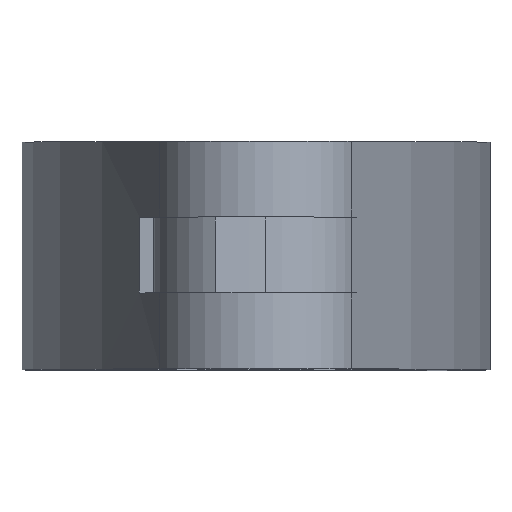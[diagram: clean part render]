
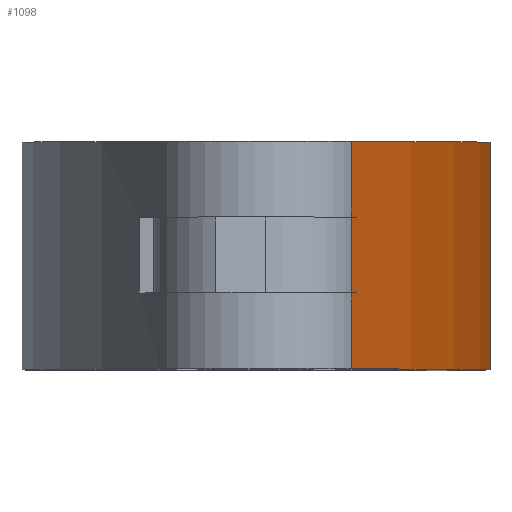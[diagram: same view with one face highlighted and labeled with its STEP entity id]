
A CAD part, top view. The second image highlights one B-rep face of the part: STEP entity #1098.
In plain terms, the highlighted cylindrical face has radius 200.536 mm (diameter 401.073 mm), a partial arc.
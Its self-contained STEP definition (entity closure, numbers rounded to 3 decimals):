
#106=FACE_OUTER_BOUND('',#176,.T.);
#176=EDGE_LOOP('',(#885,#886,#887,#888,#889,#890));
#229=LINE('',#1758,#317);
#251=LINE('',#1899,#339);
#256=LINE('',#1908,#344);
#257=LINE('',#1910,#345);
#317=VECTOR('',#1405,10.);
#339=VECTOR('',#1475,10.);
#344=VECTOR('',#1488,10.);
#345=VECTOR('',#1491,10.);
#398=CIRCLE('',#1170,200.536);
#406=CIRCLE('',#1181,200.536);
#469=VERTEX_POINT('',#1685);
#470=VERTEX_POINT('',#1687);
#479=VERTEX_POINT('',#1711);
#480=VERTEX_POINT('',#1713);
#493=VERTEX_POINT('',#1744);
#495=VERTEX_POINT('',#1752);
#573=EDGE_CURVE('',#470,#469,#398,.T.);
#586=EDGE_CURVE('',#479,#480,#406,.T.);
#608=EDGE_CURVE('',#493,#495,#229,.T.);
#641=EDGE_CURVE('',#495,#469,#251,.T.);
#646=EDGE_CURVE('',#480,#493,#256,.T.);
#647=EDGE_CURVE('',#479,#470,#257,.T.);
#885=ORIENTED_EDGE('',*,*,#586,.F.);
#886=ORIENTED_EDGE('',*,*,#647,.T.);
#887=ORIENTED_EDGE('',*,*,#573,.T.);
#888=ORIENTED_EDGE('',*,*,#641,.F.);
#889=ORIENTED_EDGE('',*,*,#608,.F.);
#890=ORIENTED_EDGE('',*,*,#646,.F.);
#1051=CYLINDRICAL_SURFACE('',#1230,200.536);
#1098=ADVANCED_FACE('',(#106),#1051,.T.);
#1170=AXIS2_PLACEMENT_3D('',#1688,#1329,#1330);
#1181=AXIS2_PLACEMENT_3D('',#1714,#1356,#1357);
#1230=AXIS2_PLACEMENT_3D('',#1909,#1489,#1490);
#1329=DIRECTION('center_axis',(0.,-1.,0.));
#1330=DIRECTION('ref_axis',(0.953,0.,-0.304));
#1356=DIRECTION('center_axis',(0.,-1.,0.));
#1357=DIRECTION('ref_axis',(0.953,0.,-0.304));
#1405=DIRECTION('',(0.,1.,0.));
#1475=DIRECTION('',(0.,1.,0.));
#1488=DIRECTION('',(0.,1.,0.));
#1489=DIRECTION('center_axis',(0.,-1.,0.));
#1490=DIRECTION('ref_axis',(0.953,0.,-0.304));
#1491=DIRECTION('',(0.,1.,0.));
#1685=CARTESIAN_POINT('',(12.652,30.,134.709));
#1687=CARTESIAN_POINT('',(21.371,30.,-9.774));
#1688=CARTESIAN_POINT('Origin',(-169.67,30.,51.202));
#1711=CARTESIAN_POINT('',(21.371,0.,-9.774));
#1713=CARTESIAN_POINT('',(12.652,0.,134.709));
#1714=CARTESIAN_POINT('Origin',(-169.67,0.,51.202));
#1744=CARTESIAN_POINT('',(12.652,10.,134.709));
#1752=CARTESIAN_POINT('',(12.652,20.,134.709));
#1758=CARTESIAN_POINT('',(12.652,0.,134.709));
#1899=CARTESIAN_POINT('',(12.652,0.,134.709));
#1908=CARTESIAN_POINT('',(12.652,0.,134.709));
#1909=CARTESIAN_POINT('Origin',(-169.67,0.,51.202));
#1910=CARTESIAN_POINT('',(21.371,0.,-9.774));
